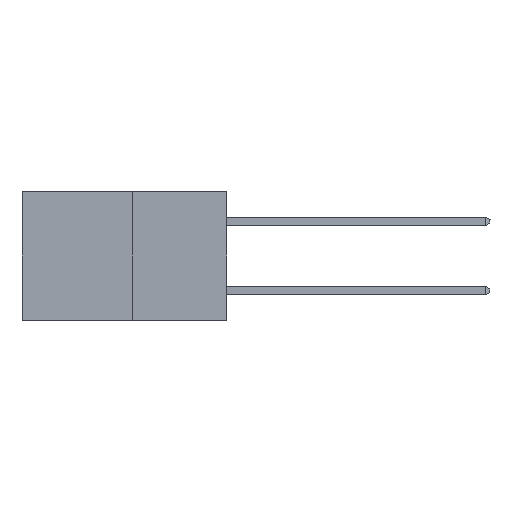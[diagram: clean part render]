
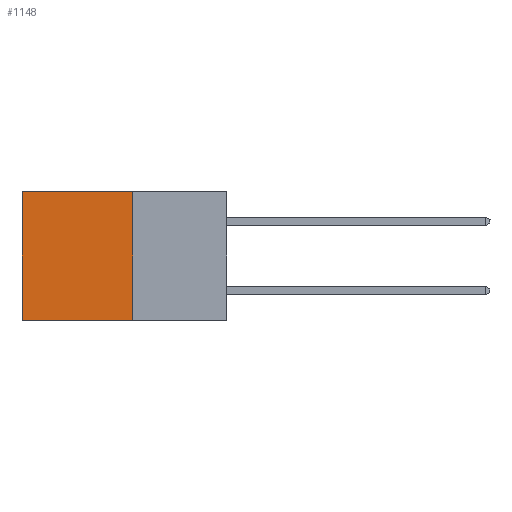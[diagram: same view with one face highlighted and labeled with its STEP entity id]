
A CAD part, left-side view. The second image highlights one B-rep face of the part: STEP entity #1148.
In plain terms, the highlighted planar face has unit normal (-1, 0, 0).
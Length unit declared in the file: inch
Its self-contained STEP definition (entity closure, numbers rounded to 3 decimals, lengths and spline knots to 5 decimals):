
#32 = CARTESIAN_POINT ( 'NONE',  ( 0.277, 0.27, 0. ) ) ;
#56 = DIRECTION ( 'NONE',  ( 0., 0., -1. ) ) ;
#977 = VERTEX_POINT ( 'NONE', #2714 ) ;
#988 = LINE ( 'NONE', #3105, #8498 ) ;
#1148 = ADVANCED_FACE ( 'NONE', ( #4768 ), #7621, .F. ) ;
#1837 = CARTESIAN_POINT ( 'NONE',  ( 0.277, 0.27, -0.37 ) ) ;
#1909 = VECTOR ( 'NONE', #8857, 39.37008 ) ;
#2017 = CARTESIAN_POINT ( 'NONE',  ( 0.277, 0.27, -0.37 ) ) ;
#2665 = LINE ( 'NONE', #4841, #4611 ) ;
#2714 = CARTESIAN_POINT ( 'NONE',  ( 0.277, 0.59, -0.37 ) ) ;
#3007 = EDGE_CURVE ( 'NONE', #6096, #9088, #7668, .T. ) ;
#3105 = CARTESIAN_POINT ( 'NONE',  ( 0.277, 0.59, -0.37 ) ) ;
#3189 = EDGE_CURVE ( 'NONE', #6096, #8988, #2665, .T. ) ;
#4034 = ORIENTED_EDGE ( 'NONE', *, *, #3189, .T. ) ;
#4060 = CARTESIAN_POINT ( 'NONE',  ( 0.277, 0.59, 0. ) ) ;
#4611 = VECTOR ( 'NONE', #5253, 39.37008 ) ;
#4707 = AXIS2_PLACEMENT_3D ( 'NONE', #6386, #8817, #7529 ) ;
#4768 = FACE_OUTER_BOUND ( 'NONE', #7392, .T. ) ;
#4841 = CARTESIAN_POINT ( 'NONE',  ( 0.277, 0.27, 0. ) ) ;
#5055 = DIRECTION ( 'NONE',  ( 0., 1., 0. ) ) ;
#5253 = DIRECTION ( 'NONE',  ( 0., 1., 0. ) ) ;
#5807 = CARTESIAN_POINT ( 'NONE',  ( 0.277, 0.27, -0.37 ) ) ;
#6096 = VERTEX_POINT ( 'NONE', #32 ) ;
#6386 = CARTESIAN_POINT ( 'NONE',  ( 0.277, 0.27, -0.37 ) ) ;
#6552 = VECTOR ( 'NONE', #5055, 39.37008 ) ;
#6564 = ORIENTED_EDGE ( 'NONE', *, *, #8721, .T. ) ;
#6593 = EDGE_CURVE ( 'NONE', #9088, #977, #8371, .T. ) ;
#7308 = ORIENTED_EDGE ( 'NONE', *, *, #3007, .F. ) ;
#7392 = EDGE_LOOP ( 'NONE', ( #6564, #8434, #7308, #4034 ) ) ;
#7529 = DIRECTION ( 'NONE',  ( 0., 0., -1. ) ) ;
#7621 = PLANE ( 'NONE',  #4707 ) ;
#7668 = LINE ( 'NONE', #1837, #1909 ) ;
#8371 = LINE ( 'NONE', #5807, #6552 ) ;
#8434 = ORIENTED_EDGE ( 'NONE', *, *, #6593, .F. ) ;
#8498 = VECTOR ( 'NONE', #56, 39.37008 ) ;
#8721 = EDGE_CURVE ( 'NONE', #8988, #977, #988, .T. ) ;
#8817 = DIRECTION ( 'NONE',  ( 1., 0., 0. ) ) ;
#8857 = DIRECTION ( 'NONE',  ( 0., 0., -1. ) ) ;
#8988 = VERTEX_POINT ( 'NONE', #4060 ) ;
#9088 = VERTEX_POINT ( 'NONE', #2017 ) ;
